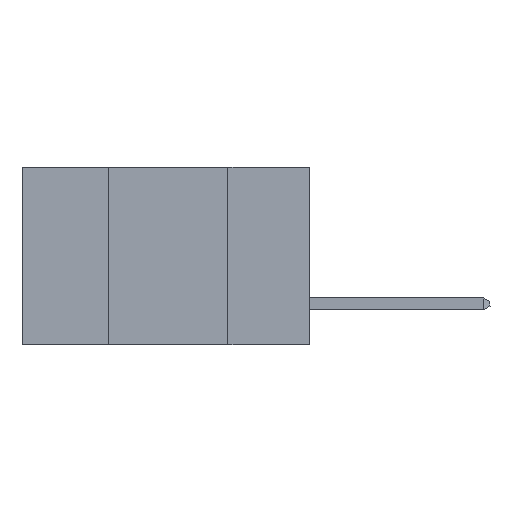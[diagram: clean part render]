
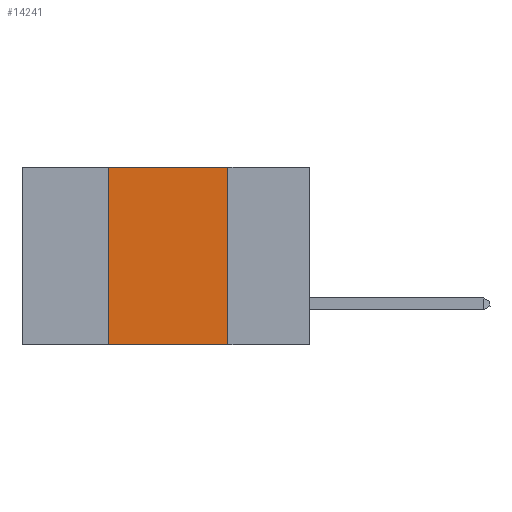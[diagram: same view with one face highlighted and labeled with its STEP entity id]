
A CAD part, left-side view. The second image highlights one B-rep face of the part: STEP entity #14241.
In plain terms, the highlighted planar face has unit normal (-1, 0, 0).
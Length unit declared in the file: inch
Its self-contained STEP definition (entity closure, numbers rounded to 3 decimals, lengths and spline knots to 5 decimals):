
#246 = FACE_OUTER_BOUND ( 'NONE', #8392, .T. ) ;
#307 = CARTESIAN_POINT ( 'NONE',  ( 0., 0.6, 0. ) ) ;
#557 = CARTESIAN_POINT ( 'NONE',  ( 0., 0.17, 0. ) ) ;
#834 = VERTEX_POINT ( 'NONE', #11685 ) ;
#1760 = DIRECTION ( 'NONE',  ( 0., 0., -1. ) ) ;
#2239 = DIRECTION ( 'NONE',  ( 0., 0., 1. ) ) ;
#2358 = EDGE_CURVE ( 'NONE', #834, #9451, #15412, .T. ) ;
#2754 = CARTESIAN_POINT ( 'NONE',  ( 0., 0.17, -0.37 ) ) ;
#3076 = VECTOR ( 'NONE', #2239, 39.37008 ) ;
#3094 = VERTEX_POINT ( 'NONE', #11373 ) ;
#4243 = VECTOR ( 'NONE', #5509, 39.37008 ) ;
#5325 = CARTESIAN_POINT ( 'NONE',  ( 0., 0.17, 0. ) ) ;
#5451 = AXIS2_PLACEMENT_3D ( 'NONE', #307, #9343, #1760 ) ;
#5509 = DIRECTION ( 'NONE',  ( 0., -1., 0. ) ) ;
#6500 = LINE ( 'NONE', #8558, #3076 ) ;
#6781 = CARTESIAN_POINT ( 'NONE',  ( 0., 0.6, -0.37 ) ) ;
#7220 = VERTEX_POINT ( 'NONE', #2754 ) ;
#7797 = DIRECTION ( 'NONE',  ( 0., -1., 0. ) ) ;
#7851 = CARTESIAN_POINT ( 'NONE',  ( 0., 0.6, 0. ) ) ;
#8392 = EDGE_LOOP ( 'NONE', ( #15255, #15584, #15875, #15904 ) ) ;
#8558 = CARTESIAN_POINT ( 'NONE',  ( 0., 0.42, 0. ) ) ;
#9343 = DIRECTION ( 'NONE',  ( 1., 0., 0. ) ) ;
#9451 = VERTEX_POINT ( 'NONE', #557 ) ;
#9796 = EDGE_CURVE ( 'NONE', #3094, #7220, #14834, .T. ) ;
#10450 = VECTOR ( 'NONE', #15119, 39.37008 ) ;
#10861 = LINE ( 'NONE', #5325, #10450 ) ;
#11373 = CARTESIAN_POINT ( 'NONE',  ( 0., 0.42, -0.37 ) ) ;
#11685 = CARTESIAN_POINT ( 'NONE',  ( 0., 0.42, 0. ) ) ;
#12226 = VECTOR ( 'NONE', #7797, 39.37008 ) ;
#12985 = PLANE ( 'NONE',  #5451 ) ;
#13876 = EDGE_CURVE ( 'NONE', #3094, #834, #6500, .T. ) ;
#14241 = ADVANCED_FACE ( 'NONE', ( #246 ), #12985, .F. ) ;
#14834 = LINE ( 'NONE', #6781, #4243 ) ;
#15119 = DIRECTION ( 'NONE',  ( 0., 0., -1. ) ) ;
#15255 = ORIENTED_EDGE ( 'NONE', *, *, #16259, .F. ) ;
#15412 = LINE ( 'NONE', #7851, #12226 ) ;
#15584 = ORIENTED_EDGE ( 'NONE', *, *, #2358, .F. ) ;
#15875 = ORIENTED_EDGE ( 'NONE', *, *, #13876, .F. ) ;
#15904 = ORIENTED_EDGE ( 'NONE', *, *, #9796, .T. ) ;
#16259 = EDGE_CURVE ( 'NONE', #9451, #7220, #10861, .T. ) ;
